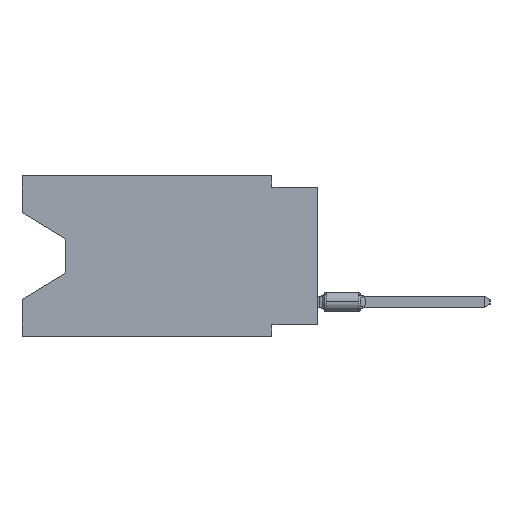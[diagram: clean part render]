
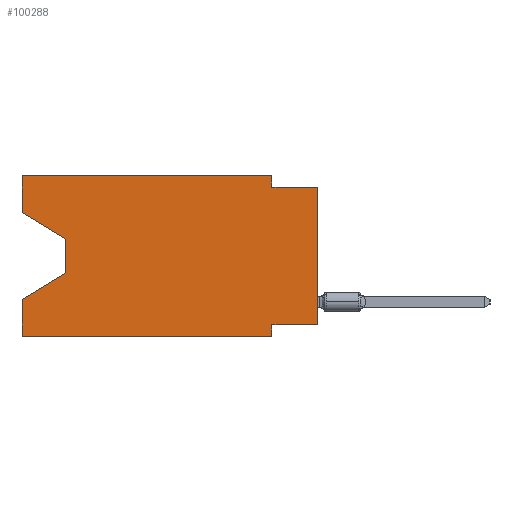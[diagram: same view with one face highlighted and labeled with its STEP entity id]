
A CAD part, left-side view. The second image highlights one B-rep face of the part: STEP entity #100288.
In plain terms, the highlighted planar face has unit normal (-1, 0, 0).
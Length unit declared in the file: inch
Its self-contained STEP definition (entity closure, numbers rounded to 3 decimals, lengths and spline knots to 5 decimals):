
#187 = VECTOR ( 'NONE', #46161, 39.37008 ) ;
#1450 = DIRECTION ( 'NONE',  ( 0., 0., -1. ) ) ;
#1608 = VECTOR ( 'NONE', #65326, 39.37008 ) ;
#1668 = PLANE ( 'NONE',  #28074 ) ;
#2603 = EDGE_CURVE ( 'NONE', #3562, #11008, #95428, .T. ) ;
#3562 = VERTEX_POINT ( 'NONE', #29578 ) ;
#3934 = VECTOR ( 'NONE', #85015, 39.37008 ) ;
#6761 = CARTESIAN_POINT ( 'NONE',  ( 0., 0.645, -0.35 ) ) ;
#7638 = LINE ( 'NONE', #38841, #39946 ) ;
#7760 = LINE ( 'NONE', #31813, #187 ) ;
#9024 = DIRECTION ( 'NONE',  ( 0., 0., -1. ) ) ;
#10960 = EDGE_LOOP ( 'NONE', ( #27029, #33198, #80875, #77516, #14068, #101022, #63156, #30505, #49833, #93476, #76768, #34717 ) ) ;
#11008 = VERTEX_POINT ( 'NONE', #75981 ) ;
#11835 = CARTESIAN_POINT ( 'NONE',  ( 0., 0.1, -0.025 ) ) ;
#12731 = CARTESIAN_POINT ( 'NONE',  ( 0., 0.645, -0.35 ) ) ;
#12869 = EDGE_CURVE ( 'NONE', #3562, #14845, #14603, .T. ) ;
#14068 = ORIENTED_EDGE ( 'NONE', *, *, #53558, .T. ) ;
#14603 = LINE ( 'NONE', #75505, #80818 ) ;
#14845 = VERTEX_POINT ( 'NONE', #54542 ) ;
#15817 = DIRECTION ( 'NONE',  ( 0., 0.855, -0.519 ) ) ;
#17044 = FACE_OUTER_BOUND ( 'NONE', #10960, .T. ) ;
#17531 = CARTESIAN_POINT ( 'NONE',  ( 0., 0.645, 0. ) ) ;
#18341 = EDGE_CURVE ( 'NONE', #11008, #42284, #70936, .T. ) ;
#22617 = LINE ( 'NONE', #6761, #3934 ) ;
#22726 = CARTESIAN_POINT ( 'NONE',  ( 0., 0.645, 0. ) ) ;
#23096 = LINE ( 'NONE', #75822, #33078 ) ;
#23928 = CARTESIAN_POINT ( 'NONE',  ( 0., 0.645, 0. ) ) ;
#24499 = VERTEX_POINT ( 'NONE', #44826 ) ;
#24552 = CARTESIAN_POINT ( 'NONE',  ( 0., 0., 0. ) ) ;
#26406 = VECTOR ( 'NONE', #71980, 39.37008 ) ;
#27029 = ORIENTED_EDGE ( 'NONE', *, *, #2603, .T. ) ;
#28074 = AXIS2_PLACEMENT_3D ( 'NONE', #17531, #47253, #86114 ) ;
#29578 = CARTESIAN_POINT ( 'NONE',  ( 0., 0.645, -0.08025 ) ) ;
#29728 = EDGE_CURVE ( 'NONE', #24499, #80627, #66662, .T. ) ;
#30505 = ORIENTED_EDGE ( 'NONE', *, *, #99422, .T. ) ;
#31813 = CARTESIAN_POINT ( 'NONE',  ( 0., 0., -0.025 ) ) ;
#32522 = CARTESIAN_POINT ( 'NONE',  ( 0., 0.645, -0.26975 ) ) ;
#32614 = EDGE_CURVE ( 'NONE', #79983, #38186, #7760, .T. ) ;
#33078 = VECTOR ( 'NONE', #1450, 39.37008 ) ;
#33085 = EDGE_CURVE ( 'NONE', #14845, #87651, #33115, .T. ) ;
#33115 = LINE ( 'NONE', #23928, #26406 ) ;
#33198 = ORIENTED_EDGE ( 'NONE', *, *, #18341, .T. ) ;
#34717 = ORIENTED_EDGE ( 'NONE', *, *, #12869, .F. ) ;
#37627 = DIRECTION ( 'NONE',  ( 0., 0., 1. ) ) ;
#38186 = VERTEX_POINT ( 'NONE', #73414 ) ;
#38281 = LINE ( 'NONE', #69485, #1608 ) ;
#38432 = LINE ( 'NONE', #24552, #90001 ) ;
#38841 = CARTESIAN_POINT ( 'NONE',  ( 0., 0.55, -0.212 ) ) ;
#39419 = DIRECTION ( 'NONE',  ( 0., 0., 1. ) ) ;
#39615 = VERTEX_POINT ( 'NONE', #32522 ) ;
#39946 = VECTOR ( 'NONE', #15817, 39.37008 ) ;
#42284 = VERTEX_POINT ( 'NONE', #44573 ) ;
#44573 = CARTESIAN_POINT ( 'NONE',  ( 0., 0.55, -0.212 ) ) ;
#44826 = CARTESIAN_POINT ( 'NONE',  ( 0., 0., -0.325 ) ) ;
#45235 = CARTESIAN_POINT ( 'NONE',  ( 0., 0.1, -0.35 ) ) ;
#46161 = DIRECTION ( 'NONE',  ( 0., -1., 0. ) ) ;
#47253 = DIRECTION ( 'NONE',  ( 1., 0., 0. ) ) ;
#47653 = EDGE_CURVE ( 'NONE', #87651, #79983, #38281, .T. ) ;
#48641 = CARTESIAN_POINT ( 'NONE',  ( 0., 0.1, 0. ) ) ;
#49833 = ORIENTED_EDGE ( 'NONE', *, *, #32614, .F. ) ;
#50306 = CARTESIAN_POINT ( 'NONE',  ( 0., 0., -0.325 ) ) ;
#53558 = EDGE_CURVE ( 'NONE', #67265, #72195, #22617, .T. ) ;
#54542 = CARTESIAN_POINT ( 'NONE',  ( 0., 0.645, 0. ) ) ;
#55192 = EDGE_CURVE ( 'NONE', #67265, #39615, #76953, .T. ) ;
#56054 = CARTESIAN_POINT ( 'NONE',  ( 0., 0.1, -0.325 ) ) ;
#56801 = VECTOR ( 'NONE', #9024, 39.37008 ) ;
#57478 = DIRECTION ( 'NONE',  ( 0., 1., 0. ) ) ;
#59341 = EDGE_CURVE ( 'NONE', #42284, #39615, #7638, .T. ) ;
#62641 = DIRECTION ( 'NONE',  ( 0., 0., 1. ) ) ;
#63156 = ORIENTED_EDGE ( 'NONE', *, *, #29728, .F. ) ;
#63273 = CARTESIAN_POINT ( 'NONE',  ( 0., 0.55, -0.138 ) ) ;
#65326 = DIRECTION ( 'NONE',  ( 0., 0., -1. ) ) ;
#66662 = LINE ( 'NONE', #50306, #70087 ) ;
#67265 = VERTEX_POINT ( 'NONE', #12731 ) ;
#69485 = CARTESIAN_POINT ( 'NONE',  ( 0., 0.1, 0. ) ) ;
#70087 = VECTOR ( 'NONE', #57478, 39.37008 ) ;
#70302 = EDGE_CURVE ( 'NONE', #80627, #72195, #23096, .T. ) ;
#70936 = LINE ( 'NONE', #63273, #56801 ) ;
#71980 = DIRECTION ( 'NONE',  ( 0., -1., 0. ) ) ;
#72195 = VERTEX_POINT ( 'NONE', #45235 ) ;
#72378 = DIRECTION ( 'NONE',  ( 0., -0.855, -0.519 ) ) ;
#73414 = CARTESIAN_POINT ( 'NONE',  ( 0., 0., -0.025 ) ) ;
#75505 = CARTESIAN_POINT ( 'NONE',  ( 0., 0.645, 0. ) ) ;
#75822 = CARTESIAN_POINT ( 'NONE',  ( 0., 0.1, -0.35 ) ) ;
#75981 = CARTESIAN_POINT ( 'NONE',  ( 0., 0.55, -0.138 ) ) ;
#76768 = ORIENTED_EDGE ( 'NONE', *, *, #33085, .F. ) ;
#76953 = LINE ( 'NONE', #22726, #83446 ) ;
#77516 = ORIENTED_EDGE ( 'NONE', *, *, #55192, .F. ) ;
#79983 = VERTEX_POINT ( 'NONE', #11835 ) ;
#80627 = VERTEX_POINT ( 'NONE', #56054 ) ;
#80818 = VECTOR ( 'NONE', #37627, 39.37008 ) ;
#80875 = ORIENTED_EDGE ( 'NONE', *, *, #59341, .T. ) ;
#83446 = VECTOR ( 'NONE', #62641, 39.37008 ) ;
#85015 = DIRECTION ( 'NONE',  ( 0., -1., 0. ) ) ;
#86114 = DIRECTION ( 'NONE',  ( 0., 0., -1. ) ) ;
#87651 = VERTEX_POINT ( 'NONE', #48641 ) ;
#90001 = VECTOR ( 'NONE', #39419, 39.37008 ) ;
#92515 = VECTOR ( 'NONE', #72378, 39.37008 ) ;
#93476 = ORIENTED_EDGE ( 'NONE', *, *, #47653, .F. ) ;
#95428 = LINE ( 'NONE', #96397, #92515 ) ;
#96397 = CARTESIAN_POINT ( 'NONE',  ( 0., 0.645, -0.08025 ) ) ;
#99422 = EDGE_CURVE ( 'NONE', #24499, #38186, #38432, .T. ) ;
#100288 = ADVANCED_FACE ( 'NONE', ( #17044 ), #1668, .F. ) ;
#101022 = ORIENTED_EDGE ( 'NONE', *, *, #70302, .F. ) ;
